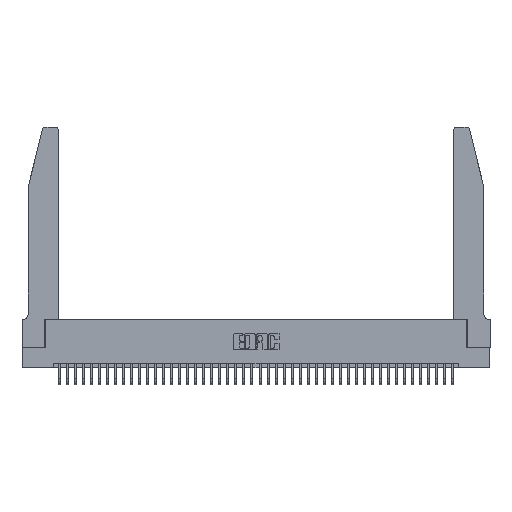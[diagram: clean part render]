
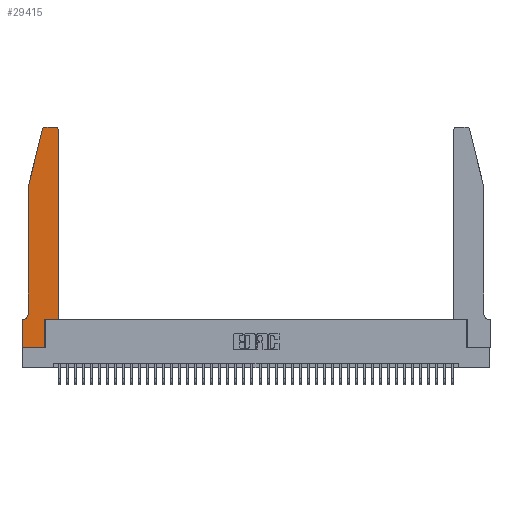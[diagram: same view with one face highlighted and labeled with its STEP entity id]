
A CAD part, top view. The second image highlights one B-rep face of the part: STEP entity #29415.
In plain terms, the highlighted planar face has unit normal (0, 0, 1).
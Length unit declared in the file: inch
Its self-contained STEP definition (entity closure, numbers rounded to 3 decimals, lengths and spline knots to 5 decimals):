
#384 = CARTESIAN_POINT ( 'NONE',  ( 0.0755, 2., 0.37 ) ) ;
#497 = VECTOR ( 'NONE', #15472, 39.37008 ) ;
#967 = CARTESIAN_POINT ( 'NONE',  ( 0.284, 2.72, 0.37 ) ) ;
#1550 = AXIS2_PLACEMENT_3D ( 'NONE', #20130, #30444, #9883 ) ;
#1964 = DIRECTION ( 'NONE',  ( 1., 0., 0. ) ) ;
#2250 = DIRECTION ( 'NONE',  ( 1., 0., 0. ) ) ;
#2335 = EDGE_LOOP ( 'NONE', ( #18659, #37162, #30972, #22319, #44271, #4000, #44062, #6480, #6072, #26485, #34634, #20165 ) ) ;
#2569 = CARTESIAN_POINT ( 'NONE',  ( 0.2865, 0.35, 0.37 ) ) ;
#2678 = EDGE_CURVE ( 'NONE', #41012, #38059, #8774, .T. ) ;
#3584 = VERTEX_POINT ( 'NONE', #38220 ) ;
#4000 = ORIENTED_EDGE ( 'NONE', *, *, #14793, .T. ) ;
#4476 = VERTEX_POINT ( 'NONE', #42030 ) ;
#4479 = DIRECTION ( 'NONE',  ( 1., 0., 0. ) ) ;
#4590 = VECTOR ( 'NONE', #2250, 39.37008 ) ;
#4749 = CARTESIAN_POINT ( 'NONE',  ( 0., 0., 0.37 ) ) ;
#4896 = DIRECTION ( 'NONE',  ( 0., -1., 0. ) ) ;
#5123 = CIRCLE ( 'NONE', #36821, 0.07 ) ;
#5910 = VERTEX_POINT ( 'NONE', #29362 ) ;
#6028 = CIRCLE ( 'NONE', #19326, 0.03 ) ;
#6072 = ORIENTED_EDGE ( 'NONE', *, *, #24621, .T. ) ;
#6390 = EDGE_CURVE ( 'NONE', #4476, #41012, #6028, .T. ) ;
#6480 = ORIENTED_EDGE ( 'NONE', *, *, #18623, .T. ) ;
#7120 = EDGE_CURVE ( 'NONE', #13171, #39277, #13096, .T. ) ;
#7694 = VECTOR ( 'NONE', #26927, 39.37008 ) ;
#8527 = VECTOR ( 'NONE', #42234, 39.37008 ) ;
#8690 = EDGE_CURVE ( 'NONE', #38059, #34402, #18859, .T. ) ;
#8774 = LINE ( 'NONE', #9779, #7694 ) ;
#9758 = LINE ( 'NONE', #12000, #497 ) ;
#9779 = CARTESIAN_POINT ( 'NONE',  ( 0.0755, 2., 0.37 ) ) ;
#9883 = DIRECTION ( 'NONE',  ( 1., 0., 0. ) ) ;
#10084 = VECTOR ( 'NONE', #12070, 39.37008 ) ;
#10687 = DIRECTION ( 'NONE',  ( 0., 0., -1. ) ) ;
#11998 = DIRECTION ( 'NONE',  ( 0., -1., 0. ) ) ;
#12000 = CARTESIAN_POINT ( 'NONE',  ( 0.0755, 0.35, 0.37 ) ) ;
#12070 = DIRECTION ( 'NONE',  ( 1., 0., 0. ) ) ;
#12248 = CARTESIAN_POINT ( 'NONE',  ( 0.2605, 2.75, 0.37 ) ) ;
#12567 = CARTESIAN_POINT ( 'NONE',  ( 0., 0., 0.37 ) ) ;
#13024 = AXIS2_PLACEMENT_3D ( 'NONE', #43136, #22648, #1964 ) ;
#13096 = CIRCLE ( 'NONE', #13024, 0.03 ) ;
#13171 = VERTEX_POINT ( 'NONE', #41043 ) ;
#13817 = LINE ( 'NONE', #12567, #4590 ) ;
#14793 = EDGE_CURVE ( 'NONE', #38870, #3584, #9758, .T. ) ;
#15002 = CARTESIAN_POINT ( 'NONE',  ( 0.4505, 0.35, 0.37 ) ) ;
#15471 = CARTESIAN_POINT ( 'NONE',  ( 0.25487, 2.72718, 0.37 ) ) ;
#15472 = DIRECTION ( 'NONE',  ( -1., 0., 0. ) ) ;
#15985 = CARTESIAN_POINT ( 'NONE',  ( 0., 0., 0.37 ) ) ;
#17692 = LINE ( 'NONE', #15002, #8527 ) ;
#18284 = LINE ( 'NONE', #4749, #35406 ) ;
#18623 = EDGE_CURVE ( 'NONE', #38906, #41413, #13817, .T. ) ;
#18659 = ORIENTED_EDGE ( 'NONE', *, *, #31068, .T. ) ;
#18859 = LINE ( 'NONE', #29093, #33819 ) ;
#19326 = AXIS2_PLACEMENT_3D ( 'NONE', #967, #25148, #4479 ) ;
#19515 = LINE ( 'NONE', #43652, #27559 ) ;
#20130 = CARTESIAN_POINT ( 'NONE',  ( 0., 0.35, 0.37 ) ) ;
#20165 = ORIENTED_EDGE ( 'NONE', *, *, #7120, .T. ) ;
#20966 = EDGE_CURVE ( 'NONE', #39278, #5910, #37455, .T. ) ;
#21437 = CARTESIAN_POINT ( 'NONE',  ( 0.2865, 0., 0.37 ) ) ;
#21795 = EDGE_CURVE ( 'NONE', #34402, #38870, #5123, .T. ) ;
#22319 = ORIENTED_EDGE ( 'NONE', *, *, #8690, .T. ) ;
#22496 = LINE ( 'NONE', #12248, #30510 ) ;
#22648 = DIRECTION ( 'NONE',  ( 0., 0., 1. ) ) ;
#24621 = EDGE_CURVE ( 'NONE', #41413, #39278, #19515, .T. ) ;
#25148 = DIRECTION ( 'NONE',  ( 0., 0., 1. ) ) ;
#26485 = ORIENTED_EDGE ( 'NONE', *, *, #20966, .T. ) ;
#26699 = CARTESIAN_POINT ( 'NONE',  ( 0.4205, 2.75, 0.37 ) ) ;
#26927 = DIRECTION ( 'NONE',  ( -0.239, -0.971, 0. ) ) ;
#27559 = VECTOR ( 'NONE', #30032, 39.37008 ) ;
#29093 = CARTESIAN_POINT ( 'NONE',  ( 0.0755, 2., 0.37 ) ) ;
#29117 = EDGE_CURVE ( 'NONE', #3584, #38906, #18284, .T. ) ;
#29362 = CARTESIAN_POINT ( 'NONE',  ( 0.4505, 0.35, 0.37 ) ) ;
#29415 = ADVANCED_FACE ( 'NONE', ( #34391 ), #30302, .T. ) ;
#30032 = DIRECTION ( 'NONE',  ( 0., 1., 0. ) ) ;
#30302 = PLANE ( 'NONE',  #1550 ) ;
#30444 = DIRECTION ( 'NONE',  ( 0., 0., 1. ) ) ;
#30510 = VECTOR ( 'NONE', #39511, 39.37008 ) ;
#30972 = ORIENTED_EDGE ( 'NONE', *, *, #2678, .T. ) ;
#31068 = EDGE_CURVE ( 'NONE', #39277, #4476, #22496, .T. ) ;
#31229 = CARTESIAN_POINT ( 'NONE',  ( 0.0055, 0.42, 0.37 ) ) ;
#32282 = EDGE_CURVE ( 'NONE', #5910, #13171, #17692, .T. ) ;
#32574 = CARTESIAN_POINT ( 'NONE',  ( 0.4505, 0.35, 0.37 ) ) ;
#33819 = VECTOR ( 'NONE', #11998, 39.37008 ) ;
#34391 = FACE_OUTER_BOUND ( 'NONE', #2335, .T. ) ;
#34402 = VERTEX_POINT ( 'NONE', #44442 ) ;
#34634 = ORIENTED_EDGE ( 'NONE', *, *, #32282, .T. ) ;
#34663 = DIRECTION ( 'NONE',  ( -1., 0., 0. ) ) ;
#35406 = VECTOR ( 'NONE', #4896, 39.37008 ) ;
#36164 = CARTESIAN_POINT ( 'NONE',  ( 0.0055, 0.35, 0.37 ) ) ;
#36821 = AXIS2_PLACEMENT_3D ( 'NONE', #31229, #10687, #34663 ) ;
#37162 = ORIENTED_EDGE ( 'NONE', *, *, #6390, .T. ) ;
#37455 = LINE ( 'NONE', #32574, #10084 ) ;
#38059 = VERTEX_POINT ( 'NONE', #384 ) ;
#38220 = CARTESIAN_POINT ( 'NONE',  ( 0., 0.35, 0.37 ) ) ;
#38870 = VERTEX_POINT ( 'NONE', #36164 ) ;
#38906 = VERTEX_POINT ( 'NONE', #15985 ) ;
#39277 = VERTEX_POINT ( 'NONE', #26699 ) ;
#39278 = VERTEX_POINT ( 'NONE', #2569 ) ;
#39511 = DIRECTION ( 'NONE',  ( -1., 0., 0. ) ) ;
#41012 = VERTEX_POINT ( 'NONE', #15471 ) ;
#41043 = CARTESIAN_POINT ( 'NONE',  ( 0.4505, 2.72, 0.37 ) ) ;
#41413 = VERTEX_POINT ( 'NONE', #21437 ) ;
#42030 = CARTESIAN_POINT ( 'NONE',  ( 0.284, 2.75, 0.37 ) ) ;
#42234 = DIRECTION ( 'NONE',  ( 0., 1., 0. ) ) ;
#43136 = CARTESIAN_POINT ( 'NONE',  ( 0.4205, 2.72, 0.37 ) ) ;
#43652 = CARTESIAN_POINT ( 'NONE',  ( 0.2865, 0.35, 0.37 ) ) ;
#44062 = ORIENTED_EDGE ( 'NONE', *, *, #29117, .T. ) ;
#44271 = ORIENTED_EDGE ( 'NONE', *, *, #21795, .T. ) ;
#44442 = CARTESIAN_POINT ( 'NONE',  ( 0.0755, 0.42, 0.37 ) ) ;
